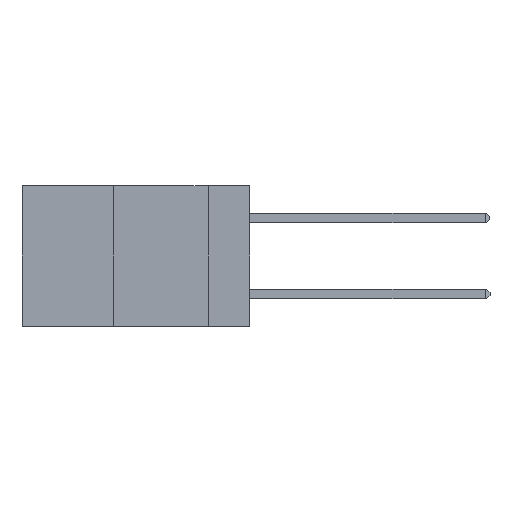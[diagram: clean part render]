
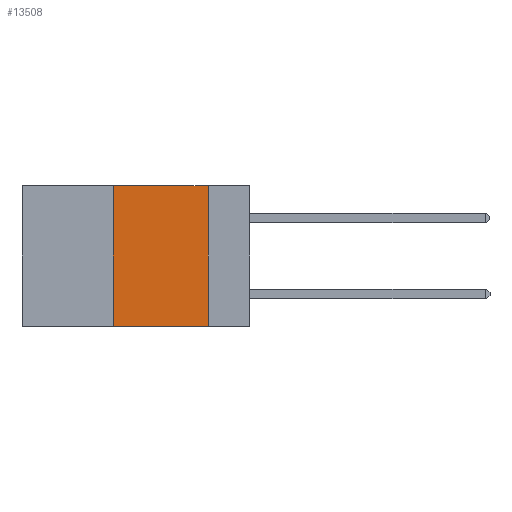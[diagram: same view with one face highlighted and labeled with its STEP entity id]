
A CAD part, left-side view. The second image highlights one B-rep face of the part: STEP entity #13508.
In plain terms, the highlighted planar face has unit normal (-1, 0, 0).
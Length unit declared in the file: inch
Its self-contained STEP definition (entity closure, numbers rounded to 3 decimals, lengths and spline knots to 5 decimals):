
#1579 = VERTEX_POINT ( 'NONE', #11700 ) ;
#1785 = EDGE_CURVE ( 'NONE', #7796, #6443, #3453, .T. ) ;
#1815 = DIRECTION ( 'NONE',  ( 0., 0., -1. ) ) ;
#3453 = LINE ( 'NONE', #10830, #12569 ) ;
#4214 = DIRECTION ( 'NONE',  ( 1., 0., 0. ) ) ;
#4482 = DIRECTION ( 'NONE',  ( 0., -1., 0. ) ) ;
#6227 = AXIS2_PLACEMENT_3D ( 'NONE', #9590, #4214, #16866 ) ;
#6443 = VERTEX_POINT ( 'NONE', #8393 ) ;
#6751 = VECTOR ( 'NONE', #19519, 39.37008 ) ;
#7796 = VERTEX_POINT ( 'NONE', #14005 ) ;
#8393 = CARTESIAN_POINT ( 'NONE',  ( 0., 0.11, -0.37 ) ) ;
#8911 = LINE ( 'NONE', #13543, #17902 ) ;
#9590 = CARTESIAN_POINT ( 'NONE',  ( 0., 0.6, 0. ) ) ;
#10632 = ORIENTED_EDGE ( 'NONE', *, *, #1785, .F. ) ;
#10830 = CARTESIAN_POINT ( 'NONE',  ( 0., 0.11, 0. ) ) ;
#11275 = VECTOR ( 'NONE', #21565, 39.37008 ) ;
#11700 = CARTESIAN_POINT ( 'NONE',  ( 0., 0.36, 0. ) ) ;
#12554 = CARTESIAN_POINT ( 'NONE',  ( 0., 0.6, 0. ) ) ;
#12569 = VECTOR ( 'NONE', #1815, 39.37008 ) ;
#13228 = FACE_OUTER_BOUND ( 'NONE', #22445, .T. ) ;
#13508 = ADVANCED_FACE ( 'NONE', ( #13228 ), #15096, .F. ) ;
#13543 = CARTESIAN_POINT ( 'NONE',  ( 0., 0.6, -0.37 ) ) ;
#14005 = CARTESIAN_POINT ( 'NONE',  ( 0., 0.11, 0. ) ) ;
#15096 = PLANE ( 'NONE',  #6227 ) ;
#15398 = ORIENTED_EDGE ( 'NONE', *, *, #22443, .F. ) ;
#16061 = LINE ( 'NONE', #19854, #11275 ) ;
#16400 = LINE ( 'NONE', #12554, #6751 ) ;
#16866 = DIRECTION ( 'NONE',  ( 0., 0., -1. ) ) ;
#17902 = VECTOR ( 'NONE', #4482, 39.37008 ) ;
#19043 = EDGE_CURVE ( 'NONE', #21928, #6443, #8911, .T. ) ;
#19519 = DIRECTION ( 'NONE',  ( 0., -1., 0. ) ) ;
#19854 = CARTESIAN_POINT ( 'NONE',  ( 0., 0.36, 0. ) ) ;
#20253 = CARTESIAN_POINT ( 'NONE',  ( 0., 0.36, -0.37 ) ) ;
#21370 = ORIENTED_EDGE ( 'NONE', *, *, #19043, .T. ) ;
#21565 = DIRECTION ( 'NONE',  ( 0., 0., 1. ) ) ;
#21674 = EDGE_CURVE ( 'NONE', #1579, #7796, #16400, .T. ) ;
#21928 = VERTEX_POINT ( 'NONE', #20253 ) ;
#22443 = EDGE_CURVE ( 'NONE', #21928, #1579, #16061, .T. ) ;
#22445 = EDGE_LOOP ( 'NONE', ( #10632, #22680, #15398, #21370 ) ) ;
#22680 = ORIENTED_EDGE ( 'NONE', *, *, #21674, .F. ) ;
